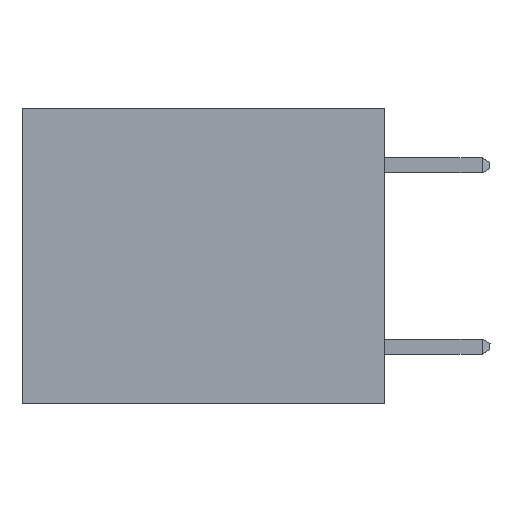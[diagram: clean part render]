
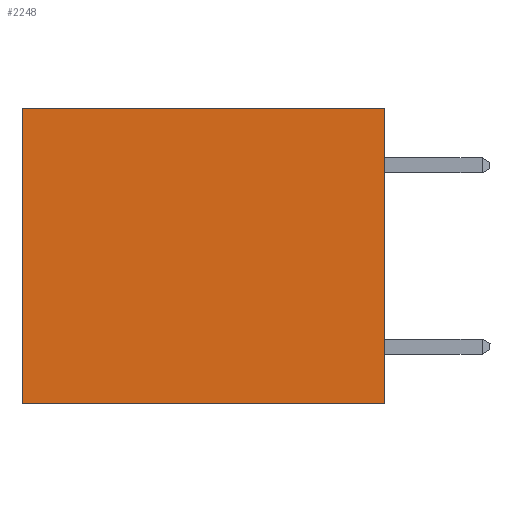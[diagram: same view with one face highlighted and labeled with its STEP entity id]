
A CAD part, left-side view. The second image highlights one B-rep face of the part: STEP entity #2248.
In plain terms, the highlighted planar face has unit normal (-1, 0, 0).
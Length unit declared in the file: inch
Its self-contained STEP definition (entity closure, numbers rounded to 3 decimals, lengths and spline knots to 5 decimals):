
#340 = LINE ( 'NONE', #6998, #18286 ) ;
#547 = EDGE_CURVE ( 'NONE', #9530, #1428, #19465, .T. ) ;
#1093 = DIRECTION ( 'NONE',  ( 1., 0., 0. ) ) ;
#1312 = VECTOR ( 'NONE', #2623, 39.37008 ) ;
#1428 = VERTEX_POINT ( 'NONE', #19053 ) ;
#2072 = DIRECTION ( 'NONE',  ( 0., 0., -1. ) ) ;
#2248 = ADVANCED_FACE ( 'NONE', ( #9423 ), #5702, .F. ) ;
#2407 = DIRECTION ( 'NONE',  ( 0., 0., -1. ) ) ;
#2623 = DIRECTION ( 'NONE',  ( 0., 0., -1. ) ) ;
#3457 = CARTESIAN_POINT ( 'NONE',  ( 0.3165, 0., -0.49 ) ) ;
#3581 = VECTOR ( 'NONE', #11557, 39.37008 ) ;
#3855 = CARTESIAN_POINT ( 'NONE',  ( 0.3165, 0., 0. ) ) ;
#4222 = EDGE_CURVE ( 'NONE', #15177, #1428, #13623, .T. ) ;
#5550 = EDGE_CURVE ( 'NONE', #16792, #15177, #340, .T. ) ;
#5702 = PLANE ( 'NONE',  #7917 ) ;
#6491 = DIRECTION ( 'NONE',  ( 0., 1., 0. ) ) ;
#6688 = EDGE_LOOP ( 'NONE', ( #11426, #14636, #14664, #15677 ) ) ;
#6998 = CARTESIAN_POINT ( 'NONE',  ( 0.3165, 0., -0.49 ) ) ;
#7917 = AXIS2_PLACEMENT_3D ( 'NONE', #18513, #1093, #2407 ) ;
#9098 = VECTOR ( 'NONE', #6491, 39.37008 ) ;
#9423 = FACE_OUTER_BOUND ( 'NONE', #6688, .T. ) ;
#9530 = VERTEX_POINT ( 'NONE', #10995 ) ;
#10982 = EDGE_CURVE ( 'NONE', #16792, #9530, #12630, .T. ) ;
#10995 = CARTESIAN_POINT ( 'NONE',  ( 0.3165, 0.6, 0. ) ) ;
#11426 = ORIENTED_EDGE ( 'NONE', *, *, #547, .T. ) ;
#11456 = CARTESIAN_POINT ( 'NONE',  ( 0.3165, 0., 0. ) ) ;
#11557 = DIRECTION ( 'NONE',  ( 0., 1., 0. ) ) ;
#12630 = LINE ( 'NONE', #11456, #9098 ) ;
#13623 = LINE ( 'NONE', #3457, #3581 ) ;
#14636 = ORIENTED_EDGE ( 'NONE', *, *, #4222, .F. ) ;
#14664 = ORIENTED_EDGE ( 'NONE', *, *, #5550, .F. ) ;
#14670 = CARTESIAN_POINT ( 'NONE',  ( 0.3165, 0., -0.49 ) ) ;
#15177 = VERTEX_POINT ( 'NONE', #14670 ) ;
#15677 = ORIENTED_EDGE ( 'NONE', *, *, #10982, .T. ) ;
#16792 = VERTEX_POINT ( 'NONE', #3855 ) ;
#18286 = VECTOR ( 'NONE', #2072, 39.37008 ) ;
#18463 = CARTESIAN_POINT ( 'NONE',  ( 0.3165, 0.6, -0.49 ) ) ;
#18513 = CARTESIAN_POINT ( 'NONE',  ( 0.3165, 0., -0.49 ) ) ;
#19053 = CARTESIAN_POINT ( 'NONE',  ( 0.3165, 0.6, -0.49 ) ) ;
#19465 = LINE ( 'NONE', #18463, #1312 ) ;
